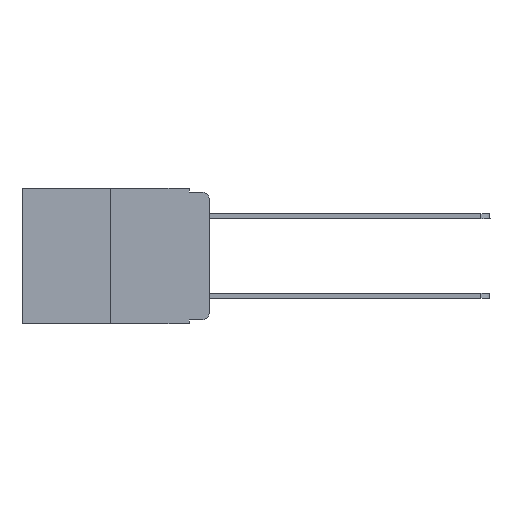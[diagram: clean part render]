
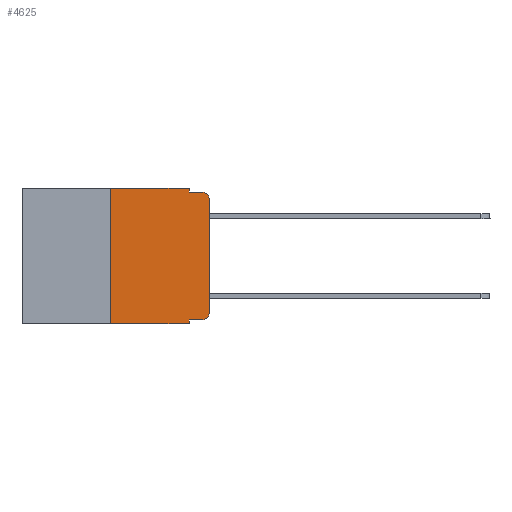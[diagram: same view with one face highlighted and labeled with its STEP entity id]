
A CAD part, left-side view. The second image highlights one B-rep face of the part: STEP entity #4625.
In plain terms, the highlighted planar face has unit normal (-1, 0, 0).
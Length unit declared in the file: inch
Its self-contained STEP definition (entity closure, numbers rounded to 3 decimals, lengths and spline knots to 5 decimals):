
#222 = CIRCLE ( 'NONE', #19462, 0.02 ) ;
#489 = FACE_OUTER_BOUND ( 'NONE', #13341, .T. ) ;
#1433 = VERTEX_POINT ( 'NONE', #20054 ) ;
#1684 = ORIENTED_EDGE ( 'NONE', *, *, #25087, .T. ) ;
#1699 = DIRECTION ( 'NONE',  ( 0., -1., 0. ) ) ;
#1728 = VERTEX_POINT ( 'NONE', #10573 ) ;
#1866 = CARTESIAN_POINT ( 'NONE',  ( 0., 0.051, -0.01 ) ) ;
#2128 = DIRECTION ( 'NONE',  ( 0., 0., -1. ) ) ;
#2632 = CIRCLE ( 'NONE', #22803, 0.02 ) ;
#2979 = ORIENTED_EDGE ( 'NONE', *, *, #7201, .F. ) ;
#3127 = EDGE_CURVE ( 'NONE', #21229, #7800, #24066, .T. ) ;
#3482 = DIRECTION ( 'NONE',  ( 0., 0., -1. ) ) ;
#3828 = LINE ( 'NONE', #16322, #5092 ) ;
#4530 = ORIENTED_EDGE ( 'NONE', *, *, #6837, .F. ) ;
#4625 = ADVANCED_FACE ( 'NONE', ( #489 ), #20751, .F. ) ;
#4762 = DIRECTION ( 'NONE',  ( 0., 0., -1. ) ) ;
#5092 = VECTOR ( 'NONE', #24516, 39.37008 ) ;
#5270 = EDGE_CURVE ( 'NONE', #23889, #17848, #6164, .T. ) ;
#6164 = LINE ( 'NONE', #7428, #10921 ) ;
#6837 = EDGE_CURVE ( 'NONE', #17505, #1433, #16428, .T. ) ;
#7073 = CARTESIAN_POINT ( 'NONE',  ( 0., 0.051, -0.343 ) ) ;
#7201 = EDGE_CURVE ( 'NONE', #21229, #23889, #14824, .T. ) ;
#7213 = VECTOR ( 'NONE', #4762, 39.37008 ) ;
#7428 = CARTESIAN_POINT ( 'NONE',  ( 0., 0.473, 0. ) ) ;
#7448 = CARTESIAN_POINT ( 'NONE',  ( 0., 0.02, -0.313 ) ) ;
#7794 = DIRECTION ( 'NONE',  ( 0., -1., 0. ) ) ;
#7800 = VERTEX_POINT ( 'NONE', #7073 ) ;
#8834 = DIRECTION ( 'NONE',  ( 0., 0., 1. ) ) ;
#9311 = LINE ( 'NONE', #17954, #24867 ) ;
#9585 = VERTEX_POINT ( 'NONE', #9634 ) ;
#9634 = CARTESIAN_POINT ( 'NONE',  ( 0., 0.02, -0.333 ) ) ;
#9816 = LINE ( 'NONE', #21207, #25358 ) ;
#10573 = CARTESIAN_POINT ( 'NONE',  ( 0., 0., -0.03 ) ) ;
#10921 = VECTOR ( 'NONE', #11185, 39.37008 ) ;
#11185 = DIRECTION ( 'NONE',  ( 0., -1., 0. ) ) ;
#11964 = CARTESIAN_POINT ( 'NONE',  ( 0., 0.25, 0. ) ) ;
#12010 = ORIENTED_EDGE ( 'NONE', *, *, #12030, .T. ) ;
#12030 = EDGE_CURVE ( 'NONE', #9585, #18718, #2632, .T. ) ;
#12454 = CARTESIAN_POINT ( 'NONE',  ( 0., 0.02, -0.03 ) ) ;
#12584 = CARTESIAN_POINT ( 'NONE',  ( 0., 0.051, -0.333 ) ) ;
#13341 = EDGE_LOOP ( 'NONE', ( #23870, #1684, #4530, #24940, #16052, #2979, #23313, #16700, #17532, #12010 ) ) ;
#13564 = LINE ( 'NONE', #16881, #7213 ) ;
#13836 = CARTESIAN_POINT ( 'NONE',  ( 0., 0.473, -0.343 ) ) ;
#13845 = EDGE_CURVE ( 'NONE', #17848, #17505, #3828, .T. ) ;
#14279 = DIRECTION ( 'NONE',  ( 1., 0., 0. ) ) ;
#14406 = CARTESIAN_POINT ( 'NONE',  ( 0., 0.25, -0.343 ) ) ;
#14448 = CARTESIAN_POINT ( 'NONE',  ( 0., 0.473, 0. ) ) ;
#14688 = CARTESIAN_POINT ( 'NONE',  ( 0., 0.25, 0. ) ) ;
#14824 = LINE ( 'NONE', #14688, #18636 ) ;
#15604 = DIRECTION ( 'NONE',  ( -1., 0., 0. ) ) ;
#16052 = ORIENTED_EDGE ( 'NONE', *, *, #5270, .F. ) ;
#16322 = CARTESIAN_POINT ( 'NONE',  ( 0., 0.051, 0. ) ) ;
#16428 = LINE ( 'NONE', #1866, #17708 ) ;
#16700 = ORIENTED_EDGE ( 'NONE', *, *, #24105, .F. ) ;
#16881 = CARTESIAN_POINT ( 'NONE',  ( 0., 0.051, 0. ) ) ;
#17505 = VERTEX_POINT ( 'NONE', #20364 ) ;
#17532 = ORIENTED_EDGE ( 'NONE', *, *, #21006, .T. ) ;
#17708 = VECTOR ( 'NONE', #1699, 39.37008 ) ;
#17848 = VERTEX_POINT ( 'NONE', #19262 ) ;
#17954 = CARTESIAN_POINT ( 'NONE',  ( 0., 0.051, -0.333 ) ) ;
#18003 = VECTOR ( 'NONE', #7794, 39.37008 ) ;
#18127 = DIRECTION ( 'NONE',  ( 0., -1., 0. ) ) ;
#18166 = VERTEX_POINT ( 'NONE', #12584 ) ;
#18636 = VECTOR ( 'NONE', #8834, 39.37008 ) ;
#18718 = VERTEX_POINT ( 'NONE', #24661 ) ;
#19262 = CARTESIAN_POINT ( 'NONE',  ( 0., 0.051, 0. ) ) ;
#19462 = AXIS2_PLACEMENT_3D ( 'NONE', #12454, #20813, #22694 ) ;
#20054 = CARTESIAN_POINT ( 'NONE',  ( 0., 0.02, -0.01 ) ) ;
#20364 = CARTESIAN_POINT ( 'NONE',  ( 0., 0.051, -0.01 ) ) ;
#20751 = PLANE ( 'NONE',  #25190 ) ;
#20813 = DIRECTION ( 'NONE',  ( -1., 0., 0. ) ) ;
#21006 = EDGE_CURVE ( 'NONE', #18166, #9585, #9311, .T. ) ;
#21207 = CARTESIAN_POINT ( 'NONE',  ( 0., 0., 0. ) ) ;
#21229 = VERTEX_POINT ( 'NONE', #14406 ) ;
#21380 = DIRECTION ( 'NONE',  ( 0., 0., 1. ) ) ;
#22694 = DIRECTION ( 'NONE',  ( 0., 0., -1. ) ) ;
#22803 = AXIS2_PLACEMENT_3D ( 'NONE', #7448, #15604, #3482 ) ;
#23313 = ORIENTED_EDGE ( 'NONE', *, *, #3127, .T. ) ;
#23458 = EDGE_CURVE ( 'NONE', #18718, #1728, #9816, .T. ) ;
#23870 = ORIENTED_EDGE ( 'NONE', *, *, #23458, .T. ) ;
#23889 = VERTEX_POINT ( 'NONE', #11964 ) ;
#24066 = LINE ( 'NONE', #13836, #18003 ) ;
#24105 = EDGE_CURVE ( 'NONE', #18166, #7800, #13564, .T. ) ;
#24516 = DIRECTION ( 'NONE',  ( 0., 0., -1. ) ) ;
#24661 = CARTESIAN_POINT ( 'NONE',  ( 0., 0., -0.313 ) ) ;
#24867 = VECTOR ( 'NONE', #18127, 39.37008 ) ;
#24940 = ORIENTED_EDGE ( 'NONE', *, *, #13845, .F. ) ;
#25087 = EDGE_CURVE ( 'NONE', #1728, #1433, #222, .T. ) ;
#25190 = AXIS2_PLACEMENT_3D ( 'NONE', #14448, #14279, #2128 ) ;
#25358 = VECTOR ( 'NONE', #21380, 39.37008 ) ;
